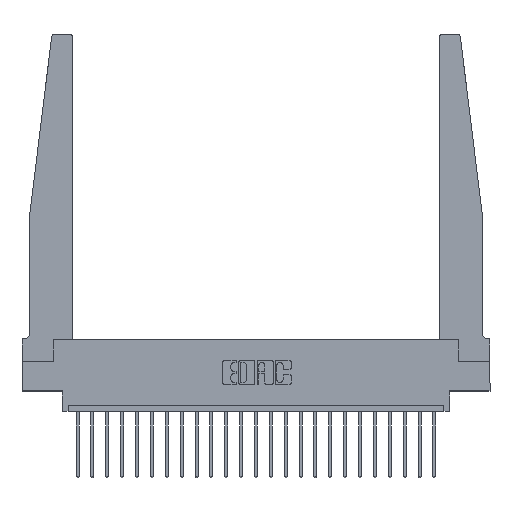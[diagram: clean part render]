
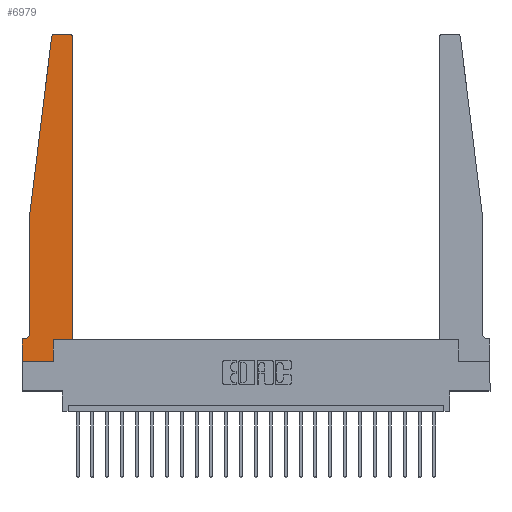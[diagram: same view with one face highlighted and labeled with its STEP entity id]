
A CAD part, top view. The second image highlights one B-rep face of the part: STEP entity #6979.
In plain terms, the highlighted planar face has unit normal (0, 0, 1).
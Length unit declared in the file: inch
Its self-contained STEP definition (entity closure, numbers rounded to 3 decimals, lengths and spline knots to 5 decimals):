
#6 = CARTESIAN_POINT ( 'NONE',  ( 0.065, 1.25, 0.37 ) ) ;
#125 = VERTEX_POINT ( 'NONE', #12398 ) ;
#268 = LINE ( 'NONE', #7439, #9133 ) ;
#557 = DIRECTION ( 'NONE',  ( 1., 0., 0. ) ) ;
#817 = LINE ( 'NONE', #7994, #10385 ) ;
#1087 = CARTESIAN_POINT ( 'NONE',  ( 0., 0.1875, 0.37 ) ) ;
#1590 = CARTESIAN_POINT ( 'NONE',  ( 0., 0., 0.37 ) ) ;
#1688 = DIRECTION ( 'NONE',  ( -1., 0., 0. ) ) ;
#2077 = CARTESIAN_POINT ( 'NONE',  ( 0.425, 0.18, 0.37 ) ) ;
#2179 = ORIENTED_EDGE ( 'NONE', *, *, #3406, .T. ) ;
#2394 = VECTOR ( 'NONE', #15839, 39.37008 ) ;
#2507 = ORIENTED_EDGE ( 'NONE', *, *, #20130, .T. ) ;
#2722 = EDGE_CURVE ( 'NONE', #17633, #21827, #5239, .T. ) ;
#3028 = AXIS2_PLACEMENT_3D ( 'NONE', #1087, #3186, #12027 ) ;
#3186 = DIRECTION ( 'NONE',  ( 0., 0., 1. ) ) ;
#3219 = EDGE_CURVE ( 'NONE', #17443, #17528, #10936, .T. ) ;
#3394 = DIRECTION ( 'NONE',  ( -0.122, -0.992, 0. ) ) ;
#3406 = EDGE_CURVE ( 'NONE', #19686, #18601, #3558, .T. ) ;
#3539 = VECTOR ( 'NONE', #557, 39.37008 ) ;
#3558 = LINE ( 'NONE', #18089, #7945 ) ;
#3643 = ORIENTED_EDGE ( 'NONE', *, *, #18299, .T. ) ;
#3867 = DIRECTION ( 'NONE',  ( 1., 0., 0. ) ) ;
#4077 = CARTESIAN_POINT ( 'NONE',  ( 0.395, 2.72, 0.37 ) ) ;
#4380 = ORIENTED_EDGE ( 'NONE', *, *, #9364, .T. ) ;
#4556 = CARTESIAN_POINT ( 'NONE',  ( 0.2605, 0.18, 0.37 ) ) ;
#4644 = DIRECTION ( 'NONE',  ( 0., 0., 1. ) ) ;
#4751 = DIRECTION ( 'NONE',  ( 0., 1., 0. ) ) ;
#5239 = CIRCLE ( 'NONE', #18317, 0.05 ) ;
#5667 = DIRECTION ( 'NONE',  ( 0., -1., 0. ) ) ;
#6201 = DIRECTION ( 'NONE',  ( -1., 0., 0. ) ) ;
#6222 = EDGE_CURVE ( 'NONE', #125, #10452, #20614, .T. ) ;
#6443 = ORIENTED_EDGE ( 'NONE', *, *, #22070, .T. ) ;
#6451 = EDGE_CURVE ( 'NONE', #13074, #12194, #15081, .T. ) ;
#6597 = PLANE ( 'NONE',  #3028 ) ;
#6870 = DIRECTION ( 'NONE',  ( 0., 0., -1. ) ) ;
#6979 = ADVANCED_FACE ( 'NONE', ( #19230 ), #6597, .T. ) ;
#7439 = CARTESIAN_POINT ( 'NONE',  ( 0., 0., 0.37 ) ) ;
#7535 = CARTESIAN_POINT ( 'NONE',  ( 0.015, 0.1875, 0.37 ) ) ;
#7945 = VECTOR ( 'NONE', #5667, 39.37008 ) ;
#7994 = CARTESIAN_POINT ( 'NONE',  ( 0.065, 0.1875, 0.37 ) ) ;
#8774 = CARTESIAN_POINT ( 'NONE',  ( 0.27653, 2.75, 0.37 ) ) ;
#9133 = VECTOR ( 'NONE', #14604, 39.37008 ) ;
#9364 = EDGE_CURVE ( 'NONE', #18601, #125, #268, .T. ) ;
#10270 = EDGE_LOOP ( 'NONE', ( #17230, #20297, #3643, #10740, #16246, #6443, #2179, #4380, #22250, #2507, #11948, #12533 ) ) ;
#10385 = VECTOR ( 'NONE', #6201, 39.37008 ) ;
#10452 = VERTEX_POINT ( 'NONE', #21460 ) ;
#10621 = CARTESIAN_POINT ( 'NONE',  ( 0.425, 2.72, 0.37 ) ) ;
#10740 = ORIENTED_EDGE ( 'NONE', *, *, #22383, .T. ) ;
#10936 = CIRCLE ( 'NONE', #11666, 0.03 ) ;
#10952 = CARTESIAN_POINT ( 'NONE',  ( 0.395, 2.75, 0.37 ) ) ;
#11102 = CARTESIAN_POINT ( 'NONE',  ( 0.24675, 2.72367, 0.37 ) ) ;
#11163 = CARTESIAN_POINT ( 'NONE',  ( 0., 0.1875, 0.37 ) ) ;
#11248 = CARTESIAN_POINT ( 'NONE',  ( 0.065, 1.25, 0.37 ) ) ;
#11479 = VECTOR ( 'NONE', #18837, 39.37008 ) ;
#11480 = LINE ( 'NONE', #11248, #20809 ) ;
#11559 = CARTESIAN_POINT ( 'NONE',  ( 0.065, 0.2375, 0.37 ) ) ;
#11594 = DIRECTION ( 'NONE',  ( 0., -1., 0. ) ) ;
#11666 = AXIS2_PLACEMENT_3D ( 'NONE', #20693, #4644, #11840 ) ;
#11715 = LINE ( 'NONE', #18678, #11954 ) ;
#11840 = DIRECTION ( 'NONE',  ( 1., 0., 0. ) ) ;
#11948 = ORIENTED_EDGE ( 'NONE', *, *, #15400, .T. ) ;
#11954 = VECTOR ( 'NONE', #4751, 39.37008 ) ;
#12027 = DIRECTION ( 'NONE',  ( 1., 0., 0. ) ) ;
#12194 = VERTEX_POINT ( 'NONE', #10952 ) ;
#12398 = CARTESIAN_POINT ( 'NONE',  ( 0.2605, 0., 0.37 ) ) ;
#12533 = ORIENTED_EDGE ( 'NONE', *, *, #6451, .T. ) ;
#12856 = AXIS2_PLACEMENT_3D ( 'NONE', #4077, #19895, #3867 ) ;
#13074 = VERTEX_POINT ( 'NONE', #10621 ) ;
#14604 = DIRECTION ( 'NONE',  ( 1., 0., 0. ) ) ;
#14930 = CARTESIAN_POINT ( 'NONE',  ( 0.425, 0.18, 0.37 ) ) ;
#15081 = CIRCLE ( 'NONE', #12856, 0.03 ) ;
#15400 = EDGE_CURVE ( 'NONE', #16186, #13074, #11715, .T. ) ;
#15839 = DIRECTION ( 'NONE',  ( -1., 0., 0. ) ) ;
#16186 = VERTEX_POINT ( 'NONE', #14930 ) ;
#16246 = ORIENTED_EDGE ( 'NONE', *, *, #2722, .T. ) ;
#17230 = ORIENTED_EDGE ( 'NONE', *, *, #19537, .T. ) ;
#17443 = VERTEX_POINT ( 'NONE', #8774 ) ;
#17528 = VERTEX_POINT ( 'NONE', #11102 ) ;
#17633 = VERTEX_POINT ( 'NONE', #11559 ) ;
#18089 = CARTESIAN_POINT ( 'NONE',  ( 0., 0., 0.37 ) ) ;
#18299 = EDGE_CURVE ( 'NONE', #17528, #21122, #20976, .T. ) ;
#18317 = AXIS2_PLACEMENT_3D ( 'NONE', #22907, #6870, #1688 ) ;
#18601 = VERTEX_POINT ( 'NONE', #1590 ) ;
#18678 = CARTESIAN_POINT ( 'NONE',  ( 0.425, 0.18, 0.37 ) ) ;
#18837 = DIRECTION ( 'NONE',  ( 0., 1., 0. ) ) ;
#19230 = FACE_OUTER_BOUND ( 'NONE', #10270, .T. ) ;
#19537 = EDGE_CURVE ( 'NONE', #12194, #17443, #20982, .T. ) ;
#19686 = VERTEX_POINT ( 'NONE', #11163 ) ;
#19895 = DIRECTION ( 'NONE',  ( 0., 0., 1. ) ) ;
#20130 = EDGE_CURVE ( 'NONE', #10452, #16186, #21868, .T. ) ;
#20297 = ORIENTED_EDGE ( 'NONE', *, *, #3219, .T. ) ;
#20614 = LINE ( 'NONE', #4556, #11479 ) ;
#20693 = CARTESIAN_POINT ( 'NONE',  ( 0.27653, 2.72, 0.37 ) ) ;
#20809 = VECTOR ( 'NONE', #11594, 39.37008 ) ;
#20976 = LINE ( 'NONE', #6, #21369 ) ;
#20982 = LINE ( 'NONE', #22972, #2394 ) ;
#21122 = VERTEX_POINT ( 'NONE', #22189 ) ;
#21369 = VECTOR ( 'NONE', #3394, 39.37008 ) ;
#21460 = CARTESIAN_POINT ( 'NONE',  ( 0.2605, 0.18, 0.37 ) ) ;
#21827 = VERTEX_POINT ( 'NONE', #7535 ) ;
#21868 = LINE ( 'NONE', #2077, #3539 ) ;
#22070 = EDGE_CURVE ( 'NONE', #21827, #19686, #817, .T. ) ;
#22189 = CARTESIAN_POINT ( 'NONE',  ( 0.065, 1.25, 0.37 ) ) ;
#22250 = ORIENTED_EDGE ( 'NONE', *, *, #6222, .T. ) ;
#22383 = EDGE_CURVE ( 'NONE', #21122, #17633, #11480, .T. ) ;
#22907 = CARTESIAN_POINT ( 'NONE',  ( 0.015, 0.2375, 0.37 ) ) ;
#22972 = CARTESIAN_POINT ( 'NONE',  ( 0.25, 2.75, 0.37 ) ) ;
